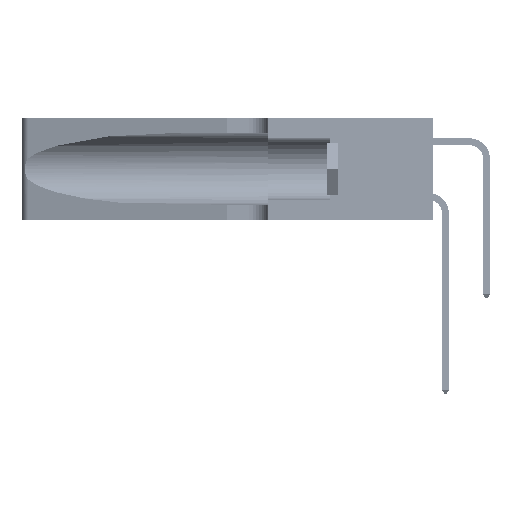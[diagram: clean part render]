
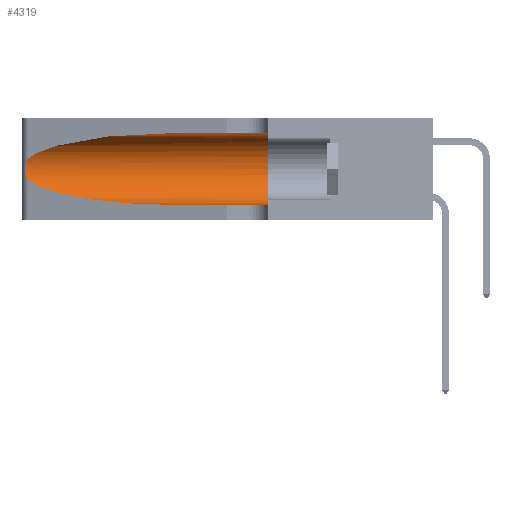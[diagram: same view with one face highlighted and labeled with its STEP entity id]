
A CAD part, left-side view. The second image highlights one B-rep face of the part: STEP entity #4319.
In plain terms, the highlighted cylindrical face has radius 3.308 mm (diameter 6.617 mm), a partial arc.
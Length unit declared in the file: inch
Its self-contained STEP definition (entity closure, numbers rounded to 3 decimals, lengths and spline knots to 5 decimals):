
#428 = EDGE_CURVE ( 'NONE', #14772, #17472, #46405, .T. ) ;
#1489 = ORIENTED_EDGE ( 'NONE', *, *, #26997, .T. ) ;
#1520 = CIRCLE ( 'NONE', #34078, 0.13025 ) ;
#1565 = VERTEX_POINT ( 'NONE', #19454 ) ;
#1645 = CARTESIAN_POINT ( 'NONE',  ( 0.1305, 1.61858, 0.31525 ) ) ;
#3692 = CARTESIAN_POINT ( 'NONE',  ( 0.25487, 1.22718, 0.22369 ) ) ;
#3722 = ORIENTED_EDGE ( 'NONE', *, *, #19446, .T. ) ;
#4313 = CARTESIAN_POINT ( 'NONE',  ( 0.1305, 0.72297, 0.31525 ) ) ;
#4319 = ADVANCED_FACE ( 'NONE', ( #38907 ), #35918, .F. ) ;
#4542 = CARTESIAN_POINT ( 'NONE',  ( 0.1305, 0.72297, 0.05475 ) ) ;
#5314 = B_SPLINE_CURVE_WITH_KNOTS ( 'NONE', 3,
 ( #16543, #38835, #31515, #12489, #47109, #24172, #16722, #43574, #10296, #43914, #8967, #40897, #17966, #39882 ),
 .UNSPECIFIED., .F., .F.,
 ( 4, 2, 2, 2, 2, 2, 4 ),
 ( 0., 0.00027, 0.00053, 0.00107, 0.0016, 0.00187, 0.00214 ),
 .UNSPECIFIED. ) ;
#5705 = CARTESIAN_POINT ( 'NONE',  ( 0.2373, 1.15595, 0.08982 ) ) ;
#6007 = DIRECTION ( 'NONE',  ( 0., -1., 0. ) ) ;
#8792 = CARTESIAN_POINT ( 'NONE',  ( 0.1305, 0.72297, 0.31525 ) ) ;
#8967 = CARTESIAN_POINT ( 'NONE',  ( 0.25789, 1.23486, 0.15765 ) ) ;
#10119 = VECTOR ( 'NONE', #16937, 39.37008 ) ;
#10296 = CARTESIAN_POINT ( 'NONE',  ( 0.26017, 1.23833, 0.17102 ) ) ;
#12223 = EDGE_CURVE ( 'NONE', #1565, #19030, #1520, .T. ) ;
#12489 = CARTESIAN_POINT ( 'NONE',  ( 0.25787, 1.23484, 0.2124 ) ) ;
#13439 = CARTESIAN_POINT ( 'NONE',  ( 0.1305, 0.72297, 0.05475 ) ) ;
#14285 = CARTESIAN_POINT ( 'NONE',  ( 0.1305, 0.35, 0.05475 ) ) ;
#14551 = ORIENTED_EDGE ( 'NONE', *, *, #37867, .T. ) ;
#14772 = VERTEX_POINT ( 'NONE', #17890 ) ;
#15750 = CARTESIAN_POINT ( 'NONE',  ( 0.18966, 0.96281, 0.31525 ) ) ;
#16543 = CARTESIAN_POINT ( 'NONE',  ( 0.25487, 1.22718, 0.22369 ) ) ;
#16722 = CARTESIAN_POINT ( 'NONE',  ( 0.26075, 1.23896, 0.19203 ) ) ;
#16937 = DIRECTION ( 'NONE',  ( 0., -1., 0. ) ) ;
#17472 = VERTEX_POINT ( 'NONE', #4542 ) ;
#17890 = CARTESIAN_POINT ( 'NONE',  ( 0.25487, 1.22718, 0.14631 ) ) ;
#17966 = CARTESIAN_POINT ( 'NONE',  ( 0.25555, 1.22993, 0.14849 ) ) ;
#19030 = VERTEX_POINT ( 'NONE', #14285 ) ;
#19446 = EDGE_CURVE ( 'NONE', #17472, #19030, #19779, .T. ) ;
#19454 = CARTESIAN_POINT ( 'NONE',  ( 0.1305, 0.35, 0.31525 ) ) ;
#19779 = LINE ( 'NONE', #43616, #10119 ) ;
#20576 = ORIENTED_EDGE ( 'NONE', *, *, #428, .T. ) ;
#20831 = AXIS2_PLACEMENT_3D ( 'NONE', #41913, #30090, #34378 ) ;
#23583 = CARTESIAN_POINT ( 'NONE',  ( 0.25487, 1.22718, 0.22369 ) ) ;
#24172 = CARTESIAN_POINT ( 'NONE',  ( 0.26018, 1.23835, 0.19895 ) ) ;
#24202 =( BOUNDED_CURVE ( )  B_SPLINE_CURVE ( 3, ( #4313, #15750, #38416, #3692 ),
 .UNSPECIFIED., .F., .F. ) 
 B_SPLINE_CURVE_WITH_KNOTS ( ( 4, 4 ),
 ( 1.5708, 2.84003 ),
 .UNSPECIFIED. ) 
 CURVE ( )  GEOMETRIC_REPRESENTATION_ITEM ( )  RATIONAL_B_SPLINE_CURVE ( ( 1., 0.87, 0.87, 1. ) ) 
 REPRESENTATION_ITEM ( '' )  );
#25984 = DIRECTION ( 'NONE',  ( 0., 1., 0. ) ) ;
#26152 = DIRECTION ( 'NONE',  ( 0., 0., 1. ) ) ;
#26997 = EDGE_CURVE ( 'NONE', #27808, #33401, #24202, .T. ) ;
#27280 = EDGE_CURVE ( 'NONE', #27808, #1565, #36517, .T. ) ;
#27808 = VERTEX_POINT ( 'NONE', #8792 ) ;
#29319 = EDGE_LOOP ( 'NONE', ( #1489, #14551, #20576, #3722, #37846, #29445 ) ) ;
#29445 = ORIENTED_EDGE ( 'NONE', *, *, #27280, .F. ) ;
#30090 = DIRECTION ( 'NONE',  ( 0., -1., 0. ) ) ;
#31515 = CARTESIAN_POINT ( 'NONE',  ( 0.25639, 1.23184, 0.21858 ) ) ;
#33401 = VERTEX_POINT ( 'NONE', #23583 ) ;
#33520 = VECTOR ( 'NONE', #6007, 39.37008 ) ;
#34078 = AXIS2_PLACEMENT_3D ( 'NONE', #45188, #25984, #26152 ) ;
#34378 = DIRECTION ( 'NONE',  ( 0., 0., -1. ) ) ;
#35918 = CYLINDRICAL_SURFACE ( 'NONE', #20831, 0.13025 ) ;
#36517 = LINE ( 'NONE', #1645, #33520 ) ;
#37846 = ORIENTED_EDGE ( 'NONE', *, *, #12223, .F. ) ;
#37867 = EDGE_CURVE ( 'NONE', #33401, #14772, #5314, .T. ) ;
#38416 = CARTESIAN_POINT ( 'NONE',  ( 0.2373, 1.15595, 0.28018 ) ) ;
#38835 = CARTESIAN_POINT ( 'NONE',  ( 0.25555, 1.22994, 0.2215 ) ) ;
#38907 = FACE_OUTER_BOUND ( 'NONE', #29319, .T. ) ;
#39803 = CARTESIAN_POINT ( 'NONE',  ( 0.18966, 0.96281, 0.05475 ) ) ;
#39882 = CARTESIAN_POINT ( 'NONE',  ( 0.25487, 1.22718, 0.14631 ) ) ;
#40897 = CARTESIAN_POINT ( 'NONE',  ( 0.25639, 1.23186, 0.15144 ) ) ;
#41913 = CARTESIAN_POINT ( 'NONE',  ( 0.1305, 1.61858, 0.185 ) ) ;
#43574 = CARTESIAN_POINT ( 'NONE',  ( 0.26075, 1.23896, 0.178 ) ) ;
#43616 = CARTESIAN_POINT ( 'NONE',  ( 0.1305, 1.61858, 0.05475 ) ) ;
#43914 = CARTESIAN_POINT ( 'NONE',  ( 0.25856, 1.23593, 0.16098 ) ) ;
#45188 = CARTESIAN_POINT ( 'NONE',  ( 0.1305, 0.35, 0.185 ) ) ;
#46405 =( BOUNDED_CURVE ( )  B_SPLINE_CURVE ( 3, ( #47696, #5705, #39803, #13439 ),
 .UNSPECIFIED., .F., .F. ) 
 B_SPLINE_CURVE_WITH_KNOTS ( ( 4, 4 ),
 ( 3.44316, 4.71239 ),
 .UNSPECIFIED. ) 
 CURVE ( )  GEOMETRIC_REPRESENTATION_ITEM ( )  RATIONAL_B_SPLINE_CURVE ( ( 1., 0.87, 0.87, 1. ) ) 
 REPRESENTATION_ITEM ( '' )  );
#47109 = CARTESIAN_POINT ( 'NONE',  ( 0.25854, 1.2359, 0.20912 ) ) ;
#47696 = CARTESIAN_POINT ( 'NONE',  ( 0.25487, 1.22718, 0.14631 ) ) ;
